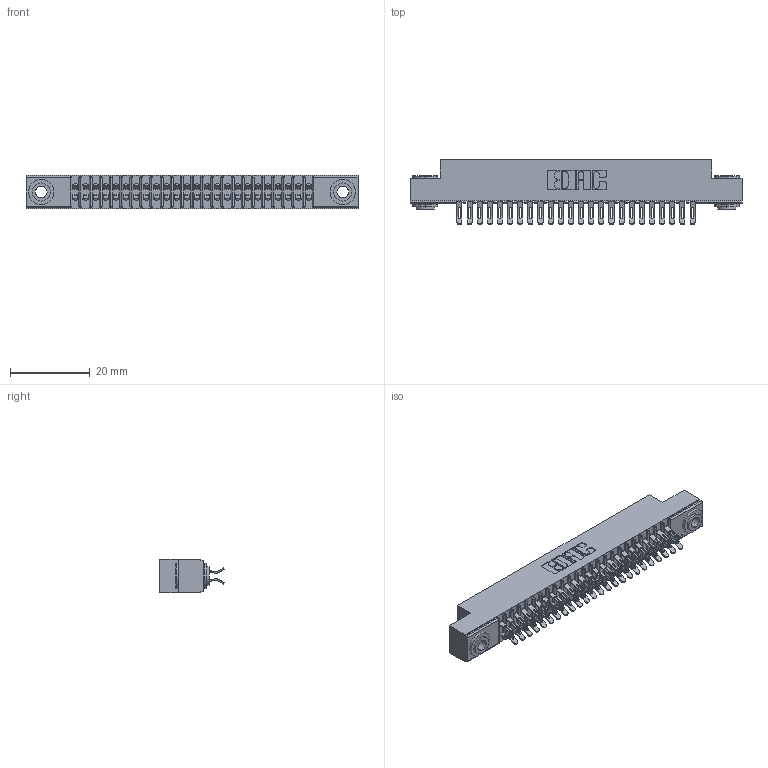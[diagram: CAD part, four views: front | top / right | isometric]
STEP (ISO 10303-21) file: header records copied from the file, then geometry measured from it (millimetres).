
FILE_DESCRIPTION (( 'STEP AP203' ), '1' );
FILE_NAME ('391-048-555-203.STEP', '2018-08-09T04:25:14', ( '' ), ( '' ), 'SwSTEP 2.0', 'SolidWorks 2016', '' );
FILE_SCHEMA (( 'CONFIG_CONTROL_DESIGN' ));
Length unit declared in the file: inch
Products named in the file (4): 341 Part_.156 (3.96) Dia Mounting Holes; 341-292-001_341-292-155; 345-250-002_345-250-002-102; 391-048-555-203
Assembly tree (51 placements, depth 2):
  391-048-555-203
    341 Part_.156 (3.96) Dia Mounting Holes
    341-292-001_341-292-155  x48
    345-250-002_345-250-002-102  x2
Bounding box: 83.19 x 16.31 x 8.38 mm (x, y, z)
Volume: 4792.7 mm3; surface area: 10721.9 mm2
Topology: 51 solids, 51 shells, 3912 faces, 11636 edges, 7574 vertices
Faces by surface type: plane 2108, cylinder 1700, sphere 50, torus 46, cone 8
Entity records: 32978 total; most frequent: CARTESIAN_POINT 5479, ORIENTED_EDGE 5424, DIRECTION 5336, EDGE_CURVE 2712, LINE 2146, VECTOR 2146, VERTEX_POINT 1722, AXIS2_PLACEMENT_3D 1595
